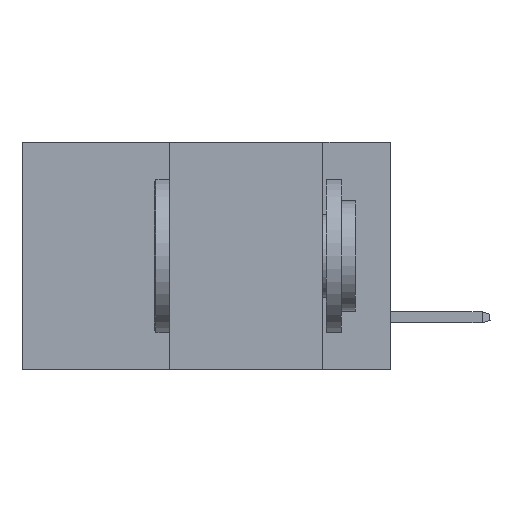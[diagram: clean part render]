
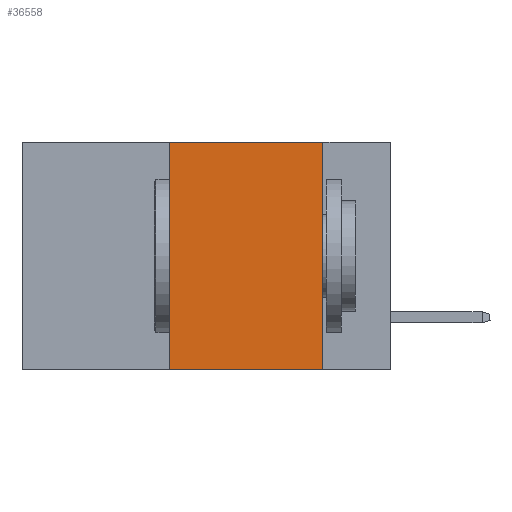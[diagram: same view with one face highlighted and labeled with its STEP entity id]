
A CAD part, left-side view. The second image highlights one B-rep face of the part: STEP entity #36558.
In plain terms, the highlighted planar face has unit normal (-1, 0, 0).
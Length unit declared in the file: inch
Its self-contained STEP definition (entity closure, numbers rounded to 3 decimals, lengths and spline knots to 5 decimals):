
#825 = CARTESIAN_POINT ( 'NONE',  ( 0., 0.36, -0.37 ) ) ;
#1785 = LINE ( 'NONE', #10046, #30062 ) ;
#2012 = VERTEX_POINT ( 'NONE', #13863 ) ;
#2470 = CARTESIAN_POINT ( 'NONE',  ( 0., 0.6, 0. ) ) ;
#2685 = VECTOR ( 'NONE', #13638, 39.37008 ) ;
#2720 = EDGE_LOOP ( 'NONE', ( #21051, #21661, #28179, #21314 ) ) ;
#3060 = CARTESIAN_POINT ( 'NONE',  ( 0., 0.36, 0. ) ) ;
#4866 = VERTEX_POINT ( 'NONE', #19724 ) ;
#8765 = LINE ( 'NONE', #2470, #27151 ) ;
#10046 = CARTESIAN_POINT ( 'NONE',  ( 0., 0.6, -0.37 ) ) ;
#10052 = DIRECTION ( 'NONE',  ( 0., 0., 1. ) ) ;
#13638 = DIRECTION ( 'NONE',  ( 0., 0., -1. ) ) ;
#13863 = CARTESIAN_POINT ( 'NONE',  ( 0., 0.11, 0. ) ) ;
#14218 = VERTEX_POINT ( 'NONE', #825 ) ;
#14505 = VECTOR ( 'NONE', #10052, 39.37008 ) ;
#16578 = EDGE_CURVE ( 'NONE', #14218, #4866, #1785, .T. ) ;
#16843 = CARTESIAN_POINT ( 'NONE',  ( 0., 0.11, 0. ) ) ;
#16976 = VERTEX_POINT ( 'NONE', #3060 ) ;
#18409 = EDGE_CURVE ( 'NONE', #14218, #16976, #39343, .T. ) ;
#19724 = CARTESIAN_POINT ( 'NONE',  ( 0., 0.11, -0.37 ) ) ;
#21051 = ORIENTED_EDGE ( 'NONE', *, *, #31273, .F. ) ;
#21072 = DIRECTION ( 'NONE',  ( 0., 0., -1. ) ) ;
#21314 = ORIENTED_EDGE ( 'NONE', *, *, #16578, .T. ) ;
#21661 = ORIENTED_EDGE ( 'NONE', *, *, #30191, .F. ) ;
#25732 = CARTESIAN_POINT ( 'NONE',  ( 0., 0.36, 0. ) ) ;
#27151 = VECTOR ( 'NONE', #31558, 39.37008 ) ;
#28179 = ORIENTED_EDGE ( 'NONE', *, *, #18409, .F. ) ;
#30062 = VECTOR ( 'NONE', #35843, 39.37008 ) ;
#30191 = EDGE_CURVE ( 'NONE', #16976, #2012, #8765, .T. ) ;
#30727 = DIRECTION ( 'NONE',  ( 1., 0., 0. ) ) ;
#30800 = FACE_OUTER_BOUND ( 'NONE', #2720, .T. ) ;
#31273 = EDGE_CURVE ( 'NONE', #2012, #4866, #34466, .T. ) ;
#31558 = DIRECTION ( 'NONE',  ( 0., -1., 0. ) ) ;
#31663 = AXIS2_PLACEMENT_3D ( 'NONE', #36996, #30727, #21072 ) ;
#33805 = PLANE ( 'NONE',  #31663 ) ;
#34466 = LINE ( 'NONE', #16843, #2685 ) ;
#35843 = DIRECTION ( 'NONE',  ( 0., -1., 0. ) ) ;
#36558 = ADVANCED_FACE ( 'NONE', ( #30800 ), #33805, .F. ) ;
#36996 = CARTESIAN_POINT ( 'NONE',  ( 0., 0.6, 0. ) ) ;
#39343 = LINE ( 'NONE', #25732, #14505 ) ;
